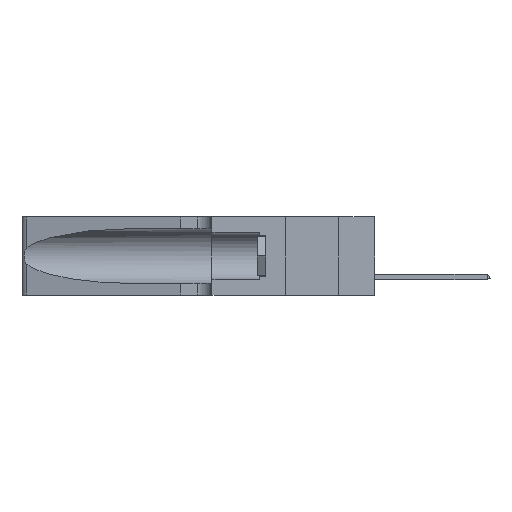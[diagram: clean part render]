
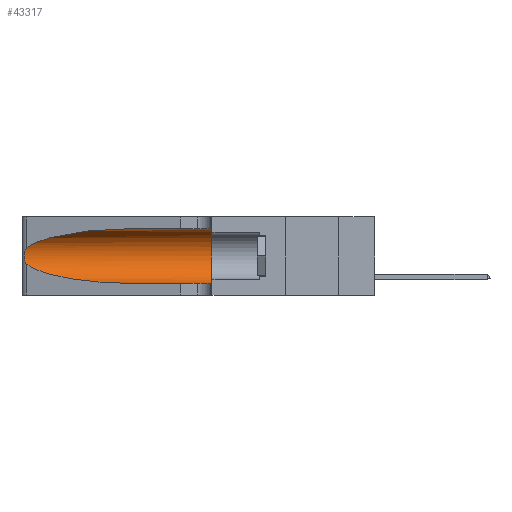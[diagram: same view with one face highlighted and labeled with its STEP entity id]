
A CAD part, left-side view. The second image highlights one B-rep face of the part: STEP entity #43317.
In plain terms, the highlighted cylindrical face has radius 3.308 mm (diameter 6.617 mm), a partial arc.
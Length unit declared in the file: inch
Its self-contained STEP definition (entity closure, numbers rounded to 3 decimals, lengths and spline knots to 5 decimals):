
#49 = DIRECTION ( 'NONE',  ( 0., 0., -1. ) ) ;
#1034 = DIRECTION ( 'NONE',  ( 0., 0., 1. ) ) ;
#2093 =( BOUNDED_CURVE ( )  B_SPLINE_CURVE ( 3, ( #43797, #32033, #24337, #20126 ),
 .UNSPECIFIED., .F., .T. ) 
 B_SPLINE_CURVE_WITH_KNOTS ( ( 4, 4 ),
 ( 3.44316, 4.71239 ),
 .UNSPECIFIED. ) 
 CURVE ( )  GEOMETRIC_REPRESENTATION_ITEM ( )  RATIONAL_B_SPLINE_CURVE ( ( 1., 0.87, 0.87, 1. ) ) 
 REPRESENTATION_ITEM ( '' )  );
#2728 = ORIENTED_EDGE ( 'NONE', *, *, #32217, .T. ) ;
#2801 = ORIENTED_EDGE ( 'NONE', *, *, #40598, .T. ) ;
#4255 = CYLINDRICAL_SURFACE ( 'NONE', #17867, 0.13025 ) ;
#4262 = VECTOR ( 'NONE', #16726, 39.37008 ) ;
#5523 = FACE_OUTER_BOUND ( 'NONE', #16111, .T. ) ;
#5713 = CARTESIAN_POINT ( 'NONE',  ( 0.25555, 1.22993, 0.14849 ) ) ;
#7478 = VERTEX_POINT ( 'NONE', #12915 ) ;
#8110 = CARTESIAN_POINT ( 'NONE',  ( 0.25487, 1.22718, 0.22369 ) ) ;
#9044 = ORIENTED_EDGE ( 'NONE', *, *, #40065, .F. ) ;
#9130 = CARTESIAN_POINT ( 'NONE',  ( 0.25487, 1.22718, 0.22369 ) ) ;
#9808 = CARTESIAN_POINT ( 'NONE',  ( 0.26075, 1.23896, 0.19203 ) ) ;
#10535 = CIRCLE ( 'NONE', #20723, 0.13025 ) ;
#10620 = ORIENTED_EDGE ( 'NONE', *, *, #34762, .T. ) ;
#11682 = DIRECTION ( 'NONE',  ( 0., -1., 0. ) ) ;
#12915 = CARTESIAN_POINT ( 'NONE',  ( 0.1305, 0.72297, 0.31525 ) ) ;
#13397 = CARTESIAN_POINT ( 'NONE',  ( 0.25787, 1.23484, 0.2124 ) ) ;
#13418 = LINE ( 'NONE', #24395, #4262 ) ;
#16111 = EDGE_LOOP ( 'NONE', ( #31762, #2728, #2801, #10620, #9044, #21858 ) ) ;
#16726 = DIRECTION ( 'NONE',  ( 0., -1., 0. ) ) ;
#16851 = CARTESIAN_POINT ( 'NONE',  ( 0.25487, 1.22718, 0.22369 ) ) ;
#17120 = CARTESIAN_POINT ( 'NONE',  ( 0.26017, 1.23833, 0.17102 ) ) ;
#17867 = AXIS2_PLACEMENT_3D ( 'NONE', #35008, #11682, #49 ) ;
#20126 = CARTESIAN_POINT ( 'NONE',  ( 0.1305, 0.72297, 0.05475 ) ) ;
#20503 = DIRECTION ( 'NONE',  ( 0., 1., 0. ) ) ;
#20723 = AXIS2_PLACEMENT_3D ( 'NONE', #39913, #20503, #1034 ) ;
#21066 = CARTESIAN_POINT ( 'NONE',  ( 0.26018, 1.23835, 0.19895 ) ) ;
#21231 = CARTESIAN_POINT ( 'NONE',  ( 0.25639, 1.23186, 0.15144 ) ) ;
#21858 = ORIENTED_EDGE ( 'NONE', *, *, #41947, .F. ) ;
#24337 = CARTESIAN_POINT ( 'NONE',  ( 0.18966, 0.96281, 0.05475 ) ) ;
#24395 = CARTESIAN_POINT ( 'NONE',  ( 0.1305, 1.61858, 0.31525 ) ) ;
#25141 = CARTESIAN_POINT ( 'NONE',  ( 0.25487, 1.22718, 0.14631 ) ) ;
#27398 = CARTESIAN_POINT ( 'NONE',  ( 0.18966, 0.96281, 0.31525 ) ) ;
#27579 = CARTESIAN_POINT ( 'NONE',  ( 0.2373, 1.15595, 0.28018 ) ) ;
#28762 = CARTESIAN_POINT ( 'NONE',  ( 0.25854, 1.2359, 0.20912 ) ) ;
#29438 = VECTOR ( 'NONE', #42883, 39.37008 ) ;
#31762 = ORIENTED_EDGE ( 'NONE', *, *, #38843, .T. ) ;
#31823 = CARTESIAN_POINT ( 'NONE',  ( 0.1305, 0.35, 0.31525 ) ) ;
#32033 = CARTESIAN_POINT ( 'NONE',  ( 0.2373, 1.15595, 0.08982 ) ) ;
#32217 = EDGE_CURVE ( 'NONE', #44032, #48900, #33949, .T. ) ;
#32903 = VERTEX_POINT ( 'NONE', #31823 ) ;
#33949 = B_SPLINE_CURVE_WITH_KNOTS ( 'NONE', 3,
 ( #9130, #48194, #44945, #13397, #28762, #21066, #9808, #40656, #17120, #48366, #44440, #21231, #5713, #25141 ),
 .UNSPECIFIED., .F., .F.,
 ( 4, 2, 2, 2, 2, 2, 4 ),
 ( 0., 0.00027, 0.00053, 0.00107, 0.0016, 0.00187, 0.00214 ),
 .UNSPECIFIED. ) ;
#34762 = EDGE_CURVE ( 'NONE', #48296, #36148, #39780, .T. ) ;
#35008 = CARTESIAN_POINT ( 'NONE',  ( 0.1305, 1.61858, 0.185 ) ) ;
#36148 = VERTEX_POINT ( 'NONE', #39337 ) ;
#38843 = EDGE_CURVE ( 'NONE', #7478, #44032, #48359, .T. ) ;
#39337 = CARTESIAN_POINT ( 'NONE',  ( 0.1305, 0.35, 0.05475 ) ) ;
#39780 = LINE ( 'NONE', #46989, #29438 ) ;
#39913 = CARTESIAN_POINT ( 'NONE',  ( 0.1305, 0.35, 0.185 ) ) ;
#40065 = EDGE_CURVE ( 'NONE', #32903, #36148, #10535, .T. ) ;
#40598 = EDGE_CURVE ( 'NONE', #48900, #48296, #2093, .T. ) ;
#40656 = CARTESIAN_POINT ( 'NONE',  ( 0.26075, 1.23896, 0.178 ) ) ;
#41947 = EDGE_CURVE ( 'NONE', #7478, #32903, #13418, .T. ) ;
#42883 = DIRECTION ( 'NONE',  ( 0., -1., 0. ) ) ;
#43317 = ADVANCED_FACE ( 'NONE', ( #5523 ), #4255, .F. ) ;
#43400 = CARTESIAN_POINT ( 'NONE',  ( 0.25487, 1.22718, 0.14631 ) ) ;
#43797 = CARTESIAN_POINT ( 'NONE',  ( 0.25487, 1.22718, 0.14631 ) ) ;
#44032 = VERTEX_POINT ( 'NONE', #16851 ) ;
#44440 = CARTESIAN_POINT ( 'NONE',  ( 0.25789, 1.23486, 0.15765 ) ) ;
#44945 = CARTESIAN_POINT ( 'NONE',  ( 0.25639, 1.23184, 0.21858 ) ) ;
#46989 = CARTESIAN_POINT ( 'NONE',  ( 0.1305, 1.61858, 0.05475 ) ) ;
#47002 = CARTESIAN_POINT ( 'NONE',  ( 0.1305, 0.72297, 0.31525 ) ) ;
#48194 = CARTESIAN_POINT ( 'NONE',  ( 0.25555, 1.22994, 0.2215 ) ) ;
#48227 = CARTESIAN_POINT ( 'NONE',  ( 0.1305, 0.72297, 0.05475 ) ) ;
#48296 = VERTEX_POINT ( 'NONE', #48227 ) ;
#48359 =( BOUNDED_CURVE ( )  B_SPLINE_CURVE ( 3, ( #47002, #27398, #27579, #8110 ),
 .UNSPECIFIED., .F., .F. ) 
 B_SPLINE_CURVE_WITH_KNOTS ( ( 4, 4 ),
 ( 1.5708, 2.84003 ),
 .UNSPECIFIED. ) 
 CURVE ( )  GEOMETRIC_REPRESENTATION_ITEM ( )  RATIONAL_B_SPLINE_CURVE ( ( 1., 0.87, 0.87, 1. ) ) 
 REPRESENTATION_ITEM ( '' )  );
#48366 = CARTESIAN_POINT ( 'NONE',  ( 0.25856, 1.23593, 0.16098 ) ) ;
#48900 = VERTEX_POINT ( 'NONE', #43400 ) ;
